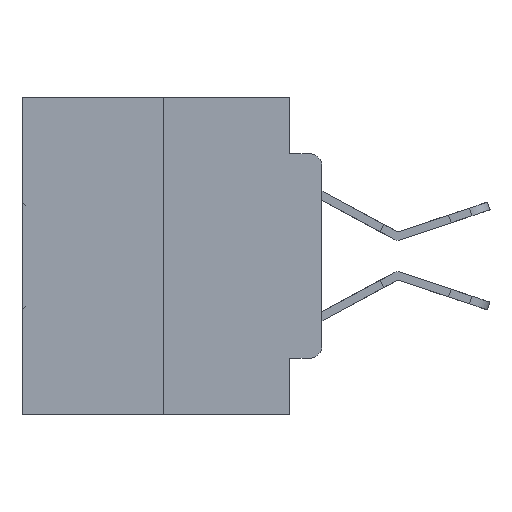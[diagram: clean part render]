
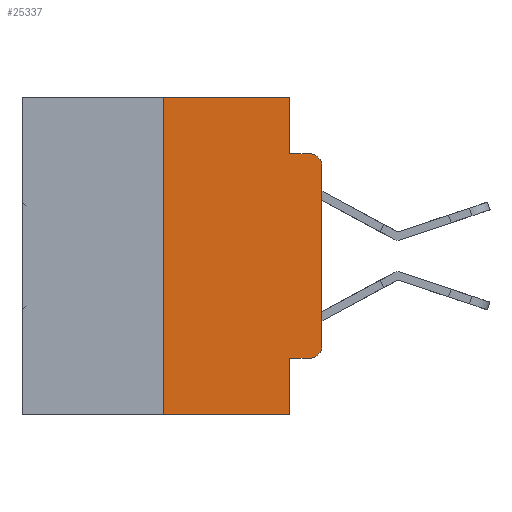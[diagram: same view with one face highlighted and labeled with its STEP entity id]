
A CAD part, left-side view. The second image highlights one B-rep face of the part: STEP entity #25337.
In plain terms, the highlighted planar face has unit normal (-1, 0, 0).
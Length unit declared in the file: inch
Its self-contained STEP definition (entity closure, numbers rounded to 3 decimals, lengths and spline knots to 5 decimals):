
#104 = CARTESIAN_POINT ( 'NONE',  ( 0., 0.051, -0.5 ) ) ;
#377 = CARTESIAN_POINT ( 'NONE',  ( 0., 0., -0.3915 ) ) ;
#927 = ORIENTED_EDGE ( 'NONE', *, *, #30449, .F. ) ;
#1389 = ORIENTED_EDGE ( 'NONE', *, *, #4934, .T. ) ;
#2084 = DIRECTION ( 'NONE',  ( 0., 0., -1. ) ) ;
#2121 = VECTOR ( 'NONE', #23744, 39.37008 ) ;
#2125 = LINE ( 'NONE', #13668, #15067 ) ;
#2259 = DIRECTION ( 'NONE',  ( 0., 0., 1. ) ) ;
#2564 = ORIENTED_EDGE ( 'NONE', *, *, #24906, .F. ) ;
#3425 = DIRECTION ( 'NONE',  ( 0., -1., 0. ) ) ;
#3483 = EDGE_CURVE ( 'NONE', #28693, #26449, #30758, .T. ) ;
#4426 = VECTOR ( 'NONE', #2259, 39.37008 ) ;
#4760 = PLANE ( 'NONE',  #7533 ) ;
#4934 = EDGE_CURVE ( 'NONE', #11967, #19478, #15871, .T. ) ;
#5290 = VERTEX_POINT ( 'NONE', #29792 ) ;
#5635 = CARTESIAN_POINT ( 'NONE',  ( 0., 0.051, 0. ) ) ;
#5783 = ORIENTED_EDGE ( 'NONE', *, *, #3483, .F. ) ;
#7059 = VECTOR ( 'NONE', #3425, 39.37008 ) ;
#7233 = CARTESIAN_POINT ( 'NONE',  ( 0., 0.051, 0. ) ) ;
#7402 = DIRECTION ( 'NONE',  ( 0., 0., -1. ) ) ;
#7533 = AXIS2_PLACEMENT_3D ( 'NONE', #15045, #22744, #7402 ) ;
#7571 = VERTEX_POINT ( 'NONE', #13625 ) ;
#7994 = LINE ( 'NONE', #27071, #27671 ) ;
#8237 = CARTESIAN_POINT ( 'NONE',  ( 0., 0.02, -0.1085 ) ) ;
#8777 = CARTESIAN_POINT ( 'NONE',  ( 0., 0.25, -0.5 ) ) ;
#9551 = AXIS2_PLACEMENT_3D ( 'NONE', #10855, #28780, #13413 ) ;
#9664 = LINE ( 'NONE', #7233, #29326 ) ;
#9883 = VERTEX_POINT ( 'NONE', #8777 ) ;
#9936 = AXIS2_PLACEMENT_3D ( 'NONE', #8237, #26213, #10857 ) ;
#10247 = CIRCLE ( 'NONE', #9936, 0.02 ) ;
#10855 = CARTESIAN_POINT ( 'NONE',  ( 0., 0.02, -0.3915 ) ) ;
#10857 = DIRECTION ( 'NONE',  ( 0., 0., -1. ) ) ;
#11141 = ORIENTED_EDGE ( 'NONE', *, *, #16249, .F. ) ;
#11967 = VERTEX_POINT ( 'NONE', #377 ) ;
#12496 = LINE ( 'NONE', #16084, #32133 ) ;
#13210 = VERTEX_POINT ( 'NONE', #28573 ) ;
#13248 = VERTEX_POINT ( 'NONE', #5635 ) ;
#13413 = DIRECTION ( 'NONE',  ( 0., 0., -1. ) ) ;
#13625 = CARTESIAN_POINT ( 'NONE',  ( 0., 0.02, -0.0885 ) ) ;
#13668 = CARTESIAN_POINT ( 'NONE',  ( 0., 0.051, -0.0885 ) ) ;
#13910 = LINE ( 'NONE', #16285, #7059 ) ;
#14072 = FACE_OUTER_BOUND ( 'NONE', #28339, .T. ) ;
#14891 = EDGE_CURVE ( 'NONE', #19478, #7571, #10247, .T. ) ;
#15045 = CARTESIAN_POINT ( 'NONE',  ( 0., 0.473, 0. ) ) ;
#15067 = VECTOR ( 'NONE', #16244, 39.37008 ) ;
#15646 = EDGE_CURVE ( 'NONE', #9883, #26449, #13910, .T. ) ;
#15871 = LINE ( 'NONE', #15906, #2121 ) ;
#15906 = CARTESIAN_POINT ( 'NONE',  ( 0., 0., 0. ) ) ;
#16084 = CARTESIAN_POINT ( 'NONE',  ( 0., 0.473, 0. ) ) ;
#16244 = DIRECTION ( 'NONE',  ( 0., -1., 0. ) ) ;
#16249 = EDGE_CURVE ( 'NONE', #28508, #7571, #2125, .T. ) ;
#16285 = CARTESIAN_POINT ( 'NONE',  ( 0., 0.473, -0.5 ) ) ;
#16721 = CARTESIAN_POINT ( 'NONE',  ( 0., 0.051, 0. ) ) ;
#16950 = CARTESIAN_POINT ( 'NONE',  ( 0., 0., -0.1085 ) ) ;
#17426 = ORIENTED_EDGE ( 'NONE', *, *, #29315, .T. ) ;
#17824 = CIRCLE ( 'NONE', #9551, 0.02 ) ;
#18608 = CARTESIAN_POINT ( 'NONE',  ( 0., 0.051, -0.4115 ) ) ;
#18974 = EDGE_CURVE ( 'NONE', #13248, #28508, #9664, .T. ) ;
#19432 = EDGE_CURVE ( 'NONE', #28693, #13210, #7994, .T. ) ;
#19478 = VERTEX_POINT ( 'NONE', #16950 ) ;
#20273 = CARTESIAN_POINT ( 'NONE',  ( 0., 0.25, 0. ) ) ;
#21058 = ORIENTED_EDGE ( 'NONE', *, *, #15646, .T. ) ;
#22567 = DIRECTION ( 'NONE',  ( 0., 0., -1. ) ) ;
#22689 = ORIENTED_EDGE ( 'NONE', *, *, #18974, .F. ) ;
#22744 = DIRECTION ( 'NONE',  ( 1., 0., 0. ) ) ;
#23523 = CARTESIAN_POINT ( 'NONE',  ( 0., 0.051, -0.0885 ) ) ;
#23744 = DIRECTION ( 'NONE',  ( 0., 0., 1. ) ) ;
#23803 = DIRECTION ( 'NONE',  ( 0., -1., 0. ) ) ;
#23933 = VECTOR ( 'NONE', #2084, 39.37008 ) ;
#24171 = LINE ( 'NONE', #20273, #4426 ) ;
#24791 = ORIENTED_EDGE ( 'NONE', *, *, #14891, .T. ) ;
#24906 = EDGE_CURVE ( 'NONE', #5290, #13248, #12496, .T. ) ;
#25337 = ADVANCED_FACE ( 'NONE', ( #14072 ), #4760, .F. ) ;
#25902 = ORIENTED_EDGE ( 'NONE', *, *, #19432, .T. ) ;
#26213 = DIRECTION ( 'NONE',  ( -1., 0., 0. ) ) ;
#26449 = VERTEX_POINT ( 'NONE', #104 ) ;
#27071 = CARTESIAN_POINT ( 'NONE',  ( 0., 0.051, -0.4115 ) ) ;
#27671 = VECTOR ( 'NONE', #29650, 39.37008 ) ;
#28339 = EDGE_LOOP ( 'NONE', ( #1389, #24791, #11141, #22689, #2564, #927, #21058, #5783, #25902, #17426 ) ) ;
#28508 = VERTEX_POINT ( 'NONE', #23523 ) ;
#28573 = CARTESIAN_POINT ( 'NONE',  ( 0., 0.02, -0.4115 ) ) ;
#28693 = VERTEX_POINT ( 'NONE', #18608 ) ;
#28780 = DIRECTION ( 'NONE',  ( -1., 0., 0. ) ) ;
#29315 = EDGE_CURVE ( 'NONE', #13210, #11967, #17824, .T. ) ;
#29326 = VECTOR ( 'NONE', #22567, 39.37008 ) ;
#29650 = DIRECTION ( 'NONE',  ( 0., -1., 0. ) ) ;
#29792 = CARTESIAN_POINT ( 'NONE',  ( 0., 0.25, 0. ) ) ;
#30449 = EDGE_CURVE ( 'NONE', #9883, #5290, #24171, .T. ) ;
#30758 = LINE ( 'NONE', #16721, #23933 ) ;
#32133 = VECTOR ( 'NONE', #23803, 39.37008 ) ;
